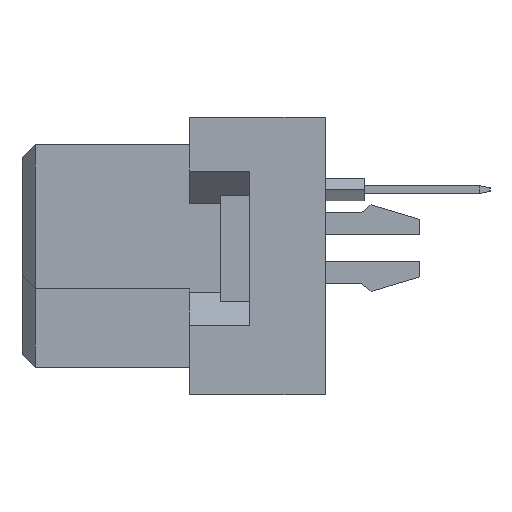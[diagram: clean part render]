
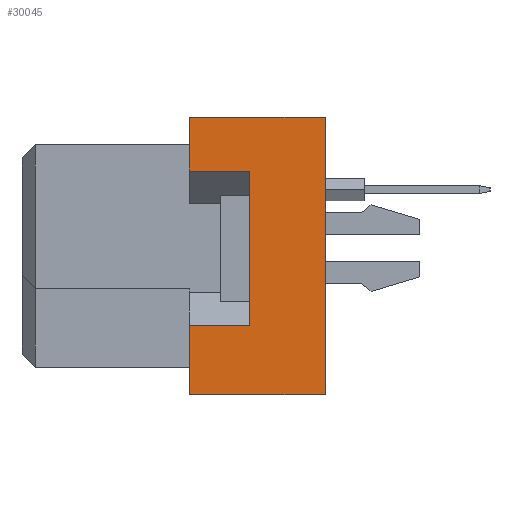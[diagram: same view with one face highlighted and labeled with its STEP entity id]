
A CAD part, left-side view. The second image highlights one B-rep face of the part: STEP entity #30045.
In plain terms, the highlighted planar face has unit normal (-1, 0, 0).
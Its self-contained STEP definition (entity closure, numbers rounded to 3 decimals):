
#283 = VERTEX_POINT ( 'NONE', #33999 ) ;
#1868 = VERTEX_POINT ( 'NONE', #29009 ) ;
#2024 = EDGE_CURVE ( 'NONE', #33842, #17993, #14375, .T. ) ;
#2371 = CARTESIAN_POINT ( 'NONE',  ( -47.5, -6.4, 5.3 ) ) ;
#4798 = VECTOR ( 'NONE', #10290, 1000. ) ;
#5785 = CARTESIAN_POINT ( 'NONE',  ( -47.5, -11.6, 5.3 ) ) ;
#6164 = CARTESIAN_POINT ( 'NONE',  ( -47.5, -11.6, 5.3 ) ) ;
#7612 = CARTESIAN_POINT ( 'NONE',  ( -47.5, -8.7, 3.25 ) ) ;
#7699 = EDGE_CURVE ( 'NONE', #31557, #1868, #37003, .T. ) ;
#9205 = CARTESIAN_POINT ( 'NONE',  ( -47.5, -6.4, -5.3 ) ) ;
#9583 = EDGE_CURVE ( 'NONE', #19067, #10588, #27540, .T. ) ;
#10290 = DIRECTION ( 'NONE',  ( 0., 1., 0. ) ) ;
#10588 = VERTEX_POINT ( 'NONE', #5785 ) ;
#10723 = CARTESIAN_POINT ( 'NONE',  ( -47.5, -11.6, -5.3 ) ) ;
#10917 = CARTESIAN_POINT ( 'NONE',  ( -47.5, -6.4, 3.25 ) ) ;
#11110 = CARTESIAN_POINT ( 'NONE',  ( -47.5, -11.6, -5.3 ) ) ;
#11708 = ORIENTED_EDGE ( 'NONE', *, *, #26574, .F. ) ;
#11792 = DIRECTION ( 'NONE',  ( 0., 0., 1. ) ) ;
#12547 = ORIENTED_EDGE ( 'NONE', *, *, #9583, .T. ) ;
#13686 = ORIENTED_EDGE ( 'NONE', *, *, #7699, .T. ) ;
#14315 = CARTESIAN_POINT ( 'NONE',  ( -47.5, -11.6, 5.3 ) ) ;
#14375 = LINE ( 'NONE', #24053, #37478 ) ;
#15176 = CARTESIAN_POINT ( 'NONE',  ( -47.5, -8.7, -2.65 ) ) ;
#15707 = VECTOR ( 'NONE', #23236, 1000. ) ;
#15977 = AXIS2_PLACEMENT_3D ( 'NONE', #14315, #28936, #23404 ) ;
#16048 = CARTESIAN_POINT ( 'NONE',  ( -47.5, -8.7, -2.65 ) ) ;
#16591 = VECTOR ( 'NONE', #34881, 1000. ) ;
#17993 = VERTEX_POINT ( 'NONE', #2371 ) ;
#18325 = ORIENTED_EDGE ( 'NONE', *, *, #33466, .F. ) ;
#19067 = VERTEX_POINT ( 'NONE', #11110 ) ;
#19166 = VECTOR ( 'NONE', #26950, 1000. ) ;
#20056 = FACE_OUTER_BOUND ( 'NONE', #20063, .T. ) ;
#20063 = EDGE_LOOP ( 'NONE', ( #13686, #34553, #11708, #12547, #37135, #25047, #30810, #18325 ) ) ;
#21617 = LINE ( 'NONE', #36267, #25246 ) ;
#23236 = DIRECTION ( 'NONE',  ( 0., 1., 0. ) ) ;
#23404 = DIRECTION ( 'NONE',  ( 0., 0., 1. ) ) ;
#24053 = CARTESIAN_POINT ( 'NONE',  ( -47.5, -6.4, -5.3 ) ) ;
#25047 = ORIENTED_EDGE ( 'NONE', *, *, #2024, .F. ) ;
#25246 = VECTOR ( 'NONE', #32890, 1000. ) ;
#25461 = VECTOR ( 'NONE', #27777, 1000. ) ;
#25684 = VERTEX_POINT ( 'NONE', #29422 ) ;
#26033 = LINE ( 'NONE', #9205, #25461 ) ;
#26072 = EDGE_CURVE ( 'NONE', #283, #33842, #37865, .T. ) ;
#26574 = EDGE_CURVE ( 'NONE', #19067, #25684, #37816, .T. ) ;
#26950 = DIRECTION ( 'NONE',  ( 0., 0., 1. ) ) ;
#27540 = LINE ( 'NONE', #6164, #19166 ) ;
#27777 = DIRECTION ( 'NONE',  ( 0., 0., 1. ) ) ;
#28936 = DIRECTION ( 'NONE',  ( -1., 0., 0. ) ) ;
#29009 = CARTESIAN_POINT ( 'NONE',  ( -47.5, -6.4, -2.65 ) ) ;
#29422 = CARTESIAN_POINT ( 'NONE',  ( -47.5, -6.4, -5.3 ) ) ;
#29531 = CARTESIAN_POINT ( 'NONE',  ( -47.5, -11.6, 5.3 ) ) ;
#30045 = ADVANCED_FACE ( 'NONE', ( #20056 ), #35462, .T. ) ;
#30810 = ORIENTED_EDGE ( 'NONE', *, *, #26072, .F. ) ;
#31557 = VERTEX_POINT ( 'NONE', #15176 ) ;
#32130 = EDGE_CURVE ( 'NONE', #10588, #17993, #32688, .T. ) ;
#32688 = LINE ( 'NONE', #29531, #16591 ) ;
#32890 = DIRECTION ( 'NONE',  ( 0., 0., 1. ) ) ;
#33466 = EDGE_CURVE ( 'NONE', #31557, #283, #21617, .T. ) ;
#33842 = VERTEX_POINT ( 'NONE', #10917 ) ;
#33999 = CARTESIAN_POINT ( 'NONE',  ( -47.5, -8.7, 3.25 ) ) ;
#34553 = ORIENTED_EDGE ( 'NONE', *, *, #37319, .F. ) ;
#34858 = DIRECTION ( 'NONE',  ( 0., 1., 0. ) ) ;
#34881 = DIRECTION ( 'NONE',  ( 0., 1., 0. ) ) ;
#35462 = PLANE ( 'NONE',  #15977 ) ;
#36267 = CARTESIAN_POINT ( 'NONE',  ( -47.5, -8.7, -2.65 ) ) ;
#37003 = LINE ( 'NONE', #16048, #4798 ) ;
#37135 = ORIENTED_EDGE ( 'NONE', *, *, #32130, .T. ) ;
#37215 = VECTOR ( 'NONE', #34858, 1000. ) ;
#37319 = EDGE_CURVE ( 'NONE', #25684, #1868, #26033, .T. ) ;
#37478 = VECTOR ( 'NONE', #11792, 1000. ) ;
#37816 = LINE ( 'NONE', #10723, #37215 ) ;
#37865 = LINE ( 'NONE', #7612, #15707 ) ;
